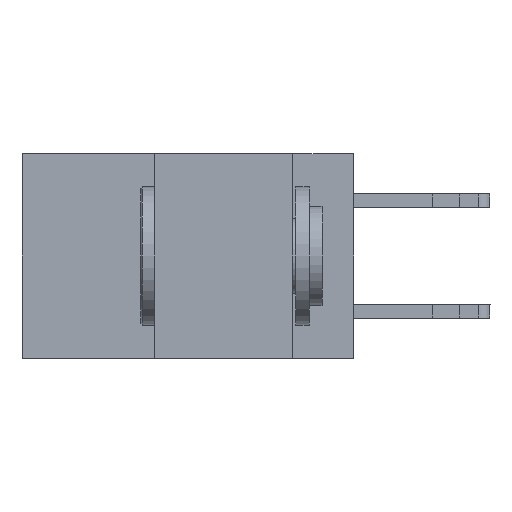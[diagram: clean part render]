
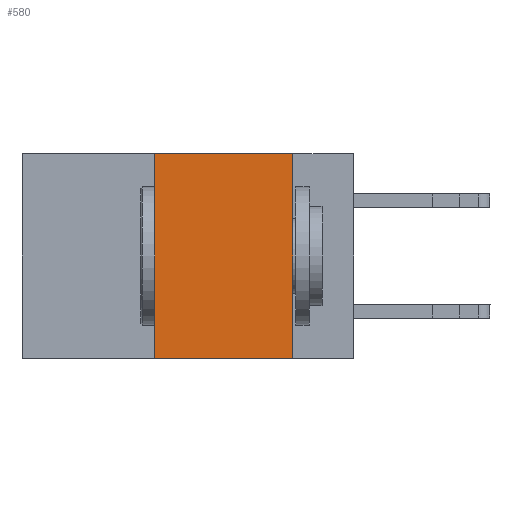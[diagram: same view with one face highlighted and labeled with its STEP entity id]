
A CAD part, left-side view. The second image highlights one B-rep face of the part: STEP entity #580.
In plain terms, the highlighted planar face has unit normal (-1, 0, 0).
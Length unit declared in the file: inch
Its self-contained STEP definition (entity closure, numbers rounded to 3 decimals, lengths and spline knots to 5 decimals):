
#580 = ADVANCED_FACE ( 'NONE', ( #13567 ), #24251, .F. ) ;
#776 = CARTESIAN_POINT ( 'NONE',  ( 0., 0.6, 0. ) ) ;
#1288 = ORIENTED_EDGE ( 'NONE', *, *, #8487, .T. ) ;
#3297 = DIRECTION ( 'NONE',  ( 0., -1., 0. ) ) ;
#3731 = CARTESIAN_POINT ( 'NONE',  ( 0., 0.11, -0.37 ) ) ;
#5676 = CARTESIAN_POINT ( 'NONE',  ( 0., 0.36, 0. ) ) ;
#5781 = VECTOR ( 'NONE', #7610, 39.37008 ) ;
#5891 = EDGE_LOOP ( 'NONE', ( #18741, #22292, #18131, #1288 ) ) ;
#5996 = CARTESIAN_POINT ( 'NONE',  ( 0., 0.6, 0. ) ) ;
#7282 = CARTESIAN_POINT ( 'NONE',  ( 0., 0.36, 0. ) ) ;
#7610 = DIRECTION ( 'NONE',  ( 0., 0., -1. ) ) ;
#8487 = EDGE_CURVE ( 'NONE', #14532, #20019, #20310, .T. ) ;
#10306 = VECTOR ( 'NONE', #3297, 39.37008 ) ;
#10348 = LINE ( 'NONE', #5996, #10306 ) ;
#11653 = CARTESIAN_POINT ( 'NONE',  ( 0., 0.11, 0. ) ) ;
#13509 = CARTESIAN_POINT ( 'NONE',  ( 0., 0.6, -0.37 ) ) ;
#13567 = FACE_OUTER_BOUND ( 'NONE', #5891, .T. ) ;
#14532 = VERTEX_POINT ( 'NONE', #24647 ) ;
#15589 = DIRECTION ( 'NONE',  ( 1., 0., 0. ) ) ;
#15842 = DIRECTION ( 'NONE',  ( 0., -1., 0. ) ) ;
#18016 = AXIS2_PLACEMENT_3D ( 'NONE', #776, #15589, #22394 ) ;
#18131 = ORIENTED_EDGE ( 'NONE', *, *, #22650, .F. ) ;
#18563 = CARTESIAN_POINT ( 'NONE',  ( 0., 0.11, 0. ) ) ;
#18741 = ORIENTED_EDGE ( 'NONE', *, *, #28234, .F. ) ;
#19123 = EDGE_CURVE ( 'NONE', #20744, #22947, #10348, .T. ) ;
#20019 = VERTEX_POINT ( 'NONE', #3731 ) ;
#20310 = LINE ( 'NONE', #13509, #24559 ) ;
#20744 = VERTEX_POINT ( 'NONE', #7282 ) ;
#20872 = VECTOR ( 'NONE', #20987, 39.37008 ) ;
#20987 = DIRECTION ( 'NONE',  ( 0., 0., 1. ) ) ;
#22292 = ORIENTED_EDGE ( 'NONE', *, *, #19123, .F. ) ;
#22394 = DIRECTION ( 'NONE',  ( 0., 0., -1. ) ) ;
#22650 = EDGE_CURVE ( 'NONE', #14532, #20744, #25450, .T. ) ;
#22947 = VERTEX_POINT ( 'NONE', #11653 ) ;
#24251 = PLANE ( 'NONE',  #18016 ) ;
#24559 = VECTOR ( 'NONE', #15842, 39.37008 ) ;
#24647 = CARTESIAN_POINT ( 'NONE',  ( 0., 0.36, -0.37 ) ) ;
#25210 = LINE ( 'NONE', #18563, #5781 ) ;
#25450 = LINE ( 'NONE', #5676, #20872 ) ;
#28234 = EDGE_CURVE ( 'NONE', #22947, #20019, #25210, .T. ) ;
